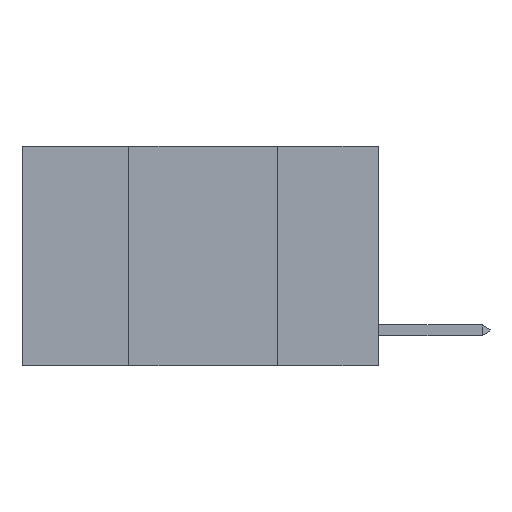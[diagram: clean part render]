
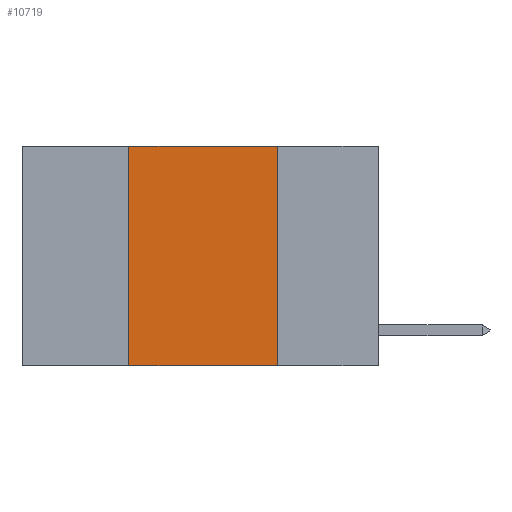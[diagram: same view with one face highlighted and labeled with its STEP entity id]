
A CAD part, left-side view. The second image highlights one B-rep face of the part: STEP entity #10719.
In plain terms, the highlighted planar face has unit normal (-1, 0, 0).
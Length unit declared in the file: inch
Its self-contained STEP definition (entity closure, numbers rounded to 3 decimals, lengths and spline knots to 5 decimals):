
#411 = DIRECTION ( 'NONE',  ( 0., -1., 0. ) ) ;
#797 = AXIS2_PLACEMENT_3D ( 'NONE', #16131, #18205, #20112 ) ;
#1040 = LINE ( 'NONE', #5386, #5402 ) ;
#1485 = EDGE_CURVE ( 'NONE', #21142, #8329, #7265, .T. ) ;
#2705 = CARTESIAN_POINT ( 'NONE',  ( 0., 0.6, -0.37 ) ) ;
#3366 = DIRECTION ( 'NONE',  ( 0., 0., 1. ) ) ;
#4995 = PLANE ( 'NONE',  #797 ) ;
#5386 = CARTESIAN_POINT ( 'NONE',  ( 0., 0.42, 0. ) ) ;
#5402 = VECTOR ( 'NONE', #3366, 39.37008 ) ;
#5726 = CARTESIAN_POINT ( 'NONE',  ( 0., 0.6, 0. ) ) ;
#7265 = LINE ( 'NONE', #2705, #12289 ) ;
#8202 = CARTESIAN_POINT ( 'NONE',  ( 0., 0.17, -0.37 ) ) ;
#8329 = VERTEX_POINT ( 'NONE', #8202 ) ;
#8390 = CARTESIAN_POINT ( 'NONE',  ( 0., 0.42, 0. ) ) ;
#9827 = VECTOR ( 'NONE', #23576, 39.37008 ) ;
#9975 = VERTEX_POINT ( 'NONE', #21470 ) ;
#10719 = ADVANCED_FACE ( 'NONE', ( #18450 ), #4995, .F. ) ;
#11853 = ORIENTED_EDGE ( 'NONE', *, *, #1485, .T. ) ;
#11939 = VECTOR ( 'NONE', #411, 39.37008 ) ;
#12289 = VECTOR ( 'NONE', #21900, 39.37008 ) ;
#12315 = CARTESIAN_POINT ( 'NONE',  ( 0., 0.17, 0. ) ) ;
#12884 = EDGE_CURVE ( 'NONE', #21142, #16345, #1040, .T. ) ;
#14149 = EDGE_LOOP ( 'NONE', ( #16375, #24151, #22689, #11853 ) ) ;
#14610 = LINE ( 'NONE', #5726, #11939 ) ;
#15827 = CARTESIAN_POINT ( 'NONE',  ( 0., 0.42, -0.37 ) ) ;
#16131 = CARTESIAN_POINT ( 'NONE',  ( 0., 0.6, 0. ) ) ;
#16345 = VERTEX_POINT ( 'NONE', #8390 ) ;
#16375 = ORIENTED_EDGE ( 'NONE', *, *, #17644, .F. ) ;
#17644 = EDGE_CURVE ( 'NONE', #9975, #8329, #19089, .T. ) ;
#18052 = EDGE_CURVE ( 'NONE', #16345, #9975, #14610, .T. ) ;
#18205 = DIRECTION ( 'NONE',  ( 1., 0., 0. ) ) ;
#18450 = FACE_OUTER_BOUND ( 'NONE', #14149, .T. ) ;
#19089 = LINE ( 'NONE', #12315, #9827 ) ;
#20112 = DIRECTION ( 'NONE',  ( 0., 0., -1. ) ) ;
#21142 = VERTEX_POINT ( 'NONE', #15827 ) ;
#21470 = CARTESIAN_POINT ( 'NONE',  ( 0., 0.17, 0. ) ) ;
#21900 = DIRECTION ( 'NONE',  ( 0., -1., 0. ) ) ;
#22689 = ORIENTED_EDGE ( 'NONE', *, *, #12884, .F. ) ;
#23576 = DIRECTION ( 'NONE',  ( 0., 0., -1. ) ) ;
#24151 = ORIENTED_EDGE ( 'NONE', *, *, #18052, .F. ) ;
